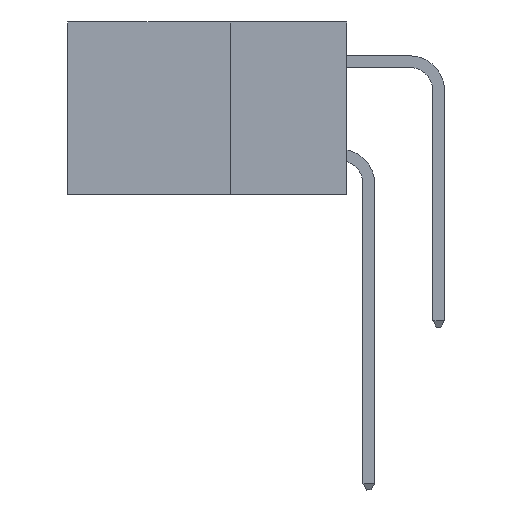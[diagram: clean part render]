
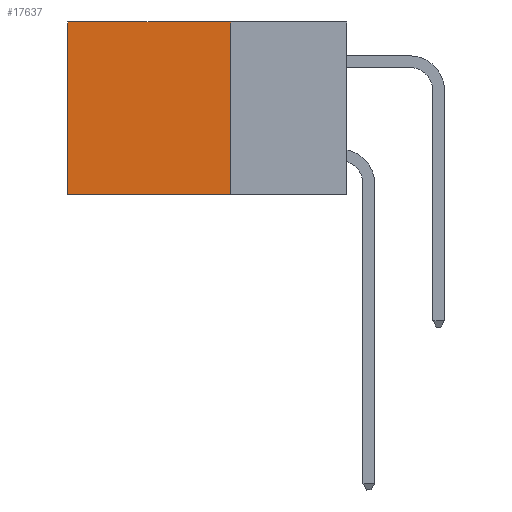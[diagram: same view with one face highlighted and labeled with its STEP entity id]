
A CAD part, left-side view. The second image highlights one B-rep face of the part: STEP entity #17637.
In plain terms, the highlighted planar face has unit normal (-1, 0, 0).
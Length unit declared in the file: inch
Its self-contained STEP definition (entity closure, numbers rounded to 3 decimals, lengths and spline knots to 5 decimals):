
#709 = ORIENTED_EDGE ( 'NONE', *, *, #8568, .F. ) ;
#1736 = LINE ( 'NONE', #16736, #5004 ) ;
#2312 = CARTESIAN_POINT ( 'NONE',  ( 0.2875, 0.25, 0. ) ) ;
#2363 = CARTESIAN_POINT ( 'NONE',  ( 0.2875, 0.25, -0.37 ) ) ;
#2424 = EDGE_CURVE ( 'NONE', #18128, #17927, #9744, .T. ) ;
#2556 = CARTESIAN_POINT ( 'NONE',  ( 0.2875, 0.6, 0. ) ) ;
#4596 = CARTESIAN_POINT ( 'NONE',  ( 0.2875, 0.25, 0. ) ) ;
#4675 = DIRECTION ( 'NONE',  ( 0., 0., -1. ) ) ;
#5004 = VECTOR ( 'NONE', #27973, 39.37008 ) ;
#7640 = CARTESIAN_POINT ( 'NONE',  ( 0.2875, 0.6, -0.37 ) ) ;
#7676 = VECTOR ( 'NONE', #21365, 39.37008 ) ;
#8568 = EDGE_CURVE ( 'NONE', #19661, #32655, #1736, .T. ) ;
#9157 = VECTOR ( 'NONE', #14354, 39.37008 ) ;
#9744 = LINE ( 'NONE', #15535, #7676 ) ;
#14354 = DIRECTION ( 'NONE',  ( 0., 1., 0. ) ) ;
#14652 = VECTOR ( 'NONE', #24643, 39.37008 ) ;
#15535 = CARTESIAN_POINT ( 'NONE',  ( 0.2875, 0.6, 0. ) ) ;
#15943 = ORIENTED_EDGE ( 'NONE', *, *, #2424, .T. ) ;
#16303 = CARTESIAN_POINT ( 'NONE',  ( 0.2875, 0.25, 0. ) ) ;
#16736 = CARTESIAN_POINT ( 'NONE',  ( 0.2875, 0.25, 0. ) ) ;
#17169 = LINE ( 'NONE', #2363, #9157 ) ;
#17637 = ADVANCED_FACE ( 'NONE', ( #27363 ), #24561, .F. ) ;
#17927 = VERTEX_POINT ( 'NONE', #7640 ) ;
#18128 = VERTEX_POINT ( 'NONE', #2556 ) ;
#19661 = VERTEX_POINT ( 'NONE', #4596 ) ;
#21365 = DIRECTION ( 'NONE',  ( 0., 0., -1. ) ) ;
#22007 = LINE ( 'NONE', #2312, #14652 ) ;
#22312 = ORIENTED_EDGE ( 'NONE', *, *, #33666, .F. ) ;
#24561 = PLANE ( 'NONE',  #35515 ) ;
#24643 = DIRECTION ( 'NONE',  ( 0., 1., 0. ) ) ;
#25096 = EDGE_LOOP ( 'NONE', ( #15943, #22312, #709, #29509 ) ) ;
#27363 = FACE_OUTER_BOUND ( 'NONE', #25096, .T. ) ;
#27973 = DIRECTION ( 'NONE',  ( 0., 0., -1. ) ) ;
#29509 = ORIENTED_EDGE ( 'NONE', *, *, #36398, .T. ) ;
#32655 = VERTEX_POINT ( 'NONE', #36009 ) ;
#33666 = EDGE_CURVE ( 'NONE', #32655, #17927, #17169, .T. ) ;
#35515 = AXIS2_PLACEMENT_3D ( 'NONE', #16303, #35978, #4675 ) ;
#35978 = DIRECTION ( 'NONE',  ( 1., 0., 0. ) ) ;
#36009 = CARTESIAN_POINT ( 'NONE',  ( 0.2875, 0.25, -0.37 ) ) ;
#36398 = EDGE_CURVE ( 'NONE', #19661, #18128, #22007, .T. ) ;
